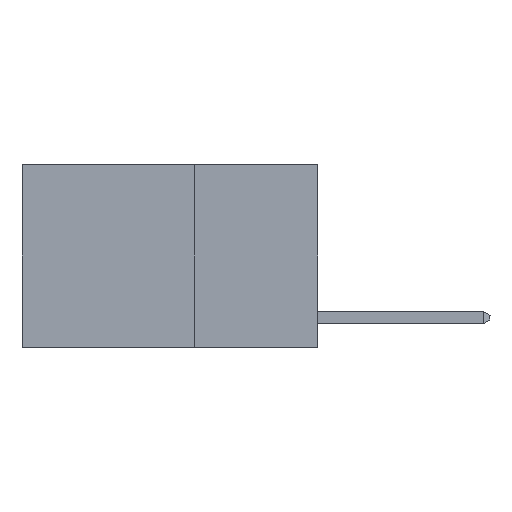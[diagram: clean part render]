
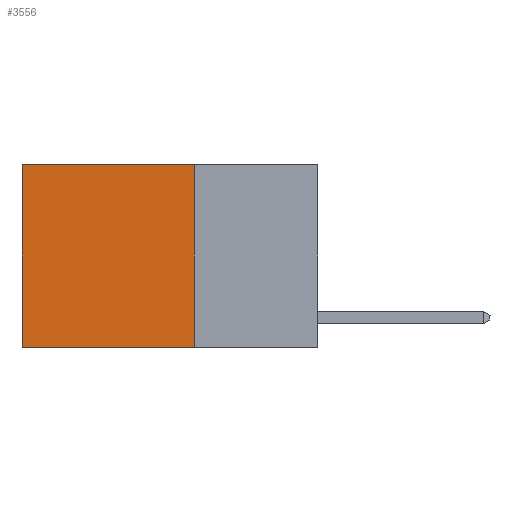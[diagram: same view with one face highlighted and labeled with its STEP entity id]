
A CAD part, left-side view. The second image highlights one B-rep face of the part: STEP entity #3556.
In plain terms, the highlighted planar face has unit normal (-1, 0, 0).
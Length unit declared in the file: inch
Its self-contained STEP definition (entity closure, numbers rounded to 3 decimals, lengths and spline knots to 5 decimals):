
#398 = CARTESIAN_POINT ( 'NONE',  ( 0.2625, 0.25, 0. ) ) ;
#936 = VECTOR ( 'NONE', #5751, 39.37008 ) ;
#1212 = CARTESIAN_POINT ( 'NONE',  ( 0.2625, 0.25, 0. ) ) ;
#1684 = EDGE_CURVE ( 'NONE', #8402, #6720, #7467, .T. ) ;
#1836 = CARTESIAN_POINT ( 'NONE',  ( 0.2625, 0.6, 0. ) ) ;
#1980 = CARTESIAN_POINT ( 'NONE',  ( 0.2625, 0.6, 0. ) ) ;
#2332 = CARTESIAN_POINT ( 'NONE',  ( 0.2625, 0.25, -0.37 ) ) ;
#2382 = VERTEX_POINT ( 'NONE', #398 ) ;
#2405 = ORIENTED_EDGE ( 'NONE', *, *, #4486, .F. ) ;
#2691 = VECTOR ( 'NONE', #6416, 39.37008 ) ;
#3045 = EDGE_LOOP ( 'NONE', ( #5121, #8278, #2405, #7001 ) ) ;
#3428 = LINE ( 'NONE', #6611, #936 ) ;
#3556 = ADVANCED_FACE ( 'NONE', ( #6717 ), #9774, .F. ) ;
#4451 = CARTESIAN_POINT ( 'NONE',  ( 0.2625, 0.25, 0. ) ) ;
#4486 = EDGE_CURVE ( 'NONE', #2382, #8402, #6698, .T. ) ;
#4833 = EDGE_CURVE ( 'NONE', #11047, #6720, #6396, .T. ) ;
#4935 = EDGE_CURVE ( 'NONE', #2382, #11047, #3428, .T. ) ;
#5121 = ORIENTED_EDGE ( 'NONE', *, *, #4833, .T. ) ;
#5389 = DIRECTION ( 'NONE',  ( 1., 0., 0. ) ) ;
#5621 = CARTESIAN_POINT ( 'NONE',  ( 0.2625, 0.6, -0.37 ) ) ;
#5751 = DIRECTION ( 'NONE',  ( 0., 1., 0. ) ) ;
#6396 = LINE ( 'NONE', #1980, #10921 ) ;
#6416 = DIRECTION ( 'NONE',  ( 0., 1., 0. ) ) ;
#6611 = CARTESIAN_POINT ( 'NONE',  ( 0.2625, 0.25, 0. ) ) ;
#6698 = LINE ( 'NONE', #1212, #11196 ) ;
#6717 = FACE_OUTER_BOUND ( 'NONE', #3045, .T. ) ;
#6720 = VERTEX_POINT ( 'NONE', #5621 ) ;
#7001 = ORIENTED_EDGE ( 'NONE', *, *, #4935, .T. ) ;
#7467 = LINE ( 'NONE', #8296, #2691 ) ;
#8278 = ORIENTED_EDGE ( 'NONE', *, *, #1684, .F. ) ;
#8296 = CARTESIAN_POINT ( 'NONE',  ( 0.2625, 0.25, -0.37 ) ) ;
#8317 = DIRECTION ( 'NONE',  ( 0., 0., -1. ) ) ;
#8402 = VERTEX_POINT ( 'NONE', #2332 ) ;
#9304 = DIRECTION ( 'NONE',  ( 0., 0., -1. ) ) ;
#9774 = PLANE ( 'NONE',  #10849 ) ;
#10849 = AXIS2_PLACEMENT_3D ( 'NONE', #4451, #5389, #11370 ) ;
#10921 = VECTOR ( 'NONE', #8317, 39.37008 ) ;
#11047 = VERTEX_POINT ( 'NONE', #1836 ) ;
#11196 = VECTOR ( 'NONE', #9304, 39.37008 ) ;
#11370 = DIRECTION ( 'NONE',  ( 0., 0., -1. ) ) ;
